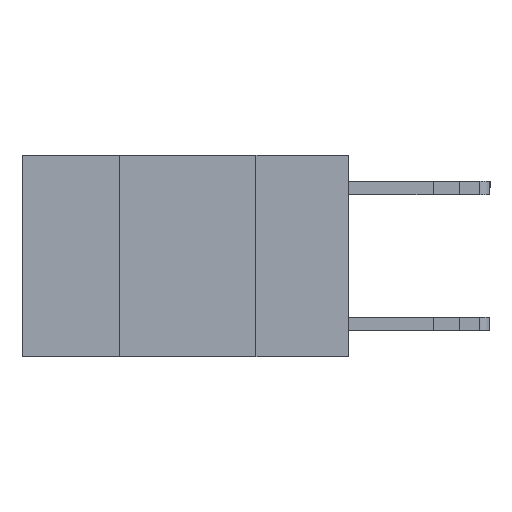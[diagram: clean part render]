
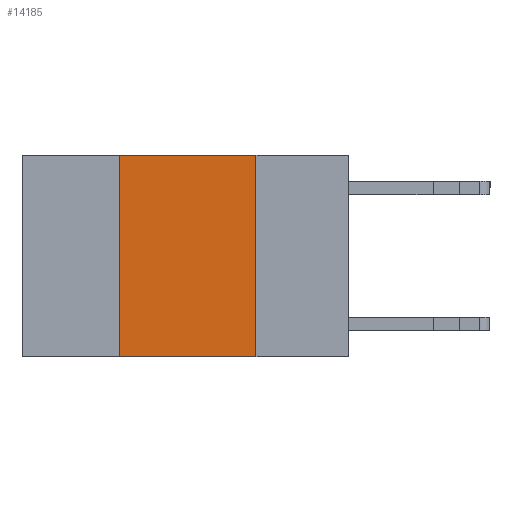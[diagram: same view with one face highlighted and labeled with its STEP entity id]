
A CAD part, left-side view. The second image highlights one B-rep face of the part: STEP entity #14185.
In plain terms, the highlighted planar face has unit normal (-1, 0, 0).
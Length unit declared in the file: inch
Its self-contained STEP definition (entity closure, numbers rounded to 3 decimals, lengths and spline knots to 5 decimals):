
#101 = EDGE_LOOP ( 'NONE', ( #18731, #4744, #9675, #9079 ) ) ;
#265 = LINE ( 'NONE', #17785, #15673 ) ;
#673 = CARTESIAN_POINT ( 'NONE',  ( 0., 0.6, -0.37 ) ) ;
#4744 = ORIENTED_EDGE ( 'NONE', *, *, #6295, .F. ) ;
#6069 = EDGE_CURVE ( 'NONE', #9672, #9356, #21163, .T. ) ;
#6085 = VECTOR ( 'NONE', #10915, 39.37008 ) ;
#6295 = EDGE_CURVE ( 'NONE', #9356, #16151, #265, .T. ) ;
#7615 = DIRECTION ( 'NONE',  ( 0., 0., -1. ) ) ;
#9074 = CARTESIAN_POINT ( 'NONE',  ( 0., 0.17, -0.37 ) ) ;
#9079 = ORIENTED_EDGE ( 'NONE', *, *, #17970, .T. ) ;
#9175 = AXIS2_PLACEMENT_3D ( 'NONE', #16132, #21436, #7615 ) ;
#9356 = VERTEX_POINT ( 'NONE', #15029 ) ;
#9433 = CARTESIAN_POINT ( 'NONE',  ( 0., 0.17, 0. ) ) ;
#9562 = VECTOR ( 'NONE', #11305, 39.37008 ) ;
#9672 = VERTEX_POINT ( 'NONE', #20808 ) ;
#9675 = ORIENTED_EDGE ( 'NONE', *, *, #6069, .F. ) ;
#9793 = VERTEX_POINT ( 'NONE', #9074 ) ;
#10817 = LINE ( 'NONE', #673, #6085 ) ;
#10915 = DIRECTION ( 'NONE',  ( 0., -1., 0. ) ) ;
#11305 = DIRECTION ( 'NONE',  ( 0., 0., 1. ) ) ;
#12551 = EDGE_CURVE ( 'NONE', #16151, #9793, #18272, .T. ) ;
#12754 = CARTESIAN_POINT ( 'NONE',  ( 0., 0.42, 0. ) ) ;
#12921 = FACE_OUTER_BOUND ( 'NONE', #101, .T. ) ;
#13404 = VECTOR ( 'NONE', #21593, 39.37008 ) ;
#14185 = ADVANCED_FACE ( 'NONE', ( #12921 ), #14686, .F. ) ;
#14686 = PLANE ( 'NONE',  #9175 ) ;
#15029 = CARTESIAN_POINT ( 'NONE',  ( 0., 0.42, 0. ) ) ;
#15673 = VECTOR ( 'NONE', #19566, 39.37008 ) ;
#16132 = CARTESIAN_POINT ( 'NONE',  ( 0., 0.6, 0. ) ) ;
#16151 = VERTEX_POINT ( 'NONE', #17762 ) ;
#17762 = CARTESIAN_POINT ( 'NONE',  ( 0., 0.17, 0. ) ) ;
#17785 = CARTESIAN_POINT ( 'NONE',  ( 0., 0.6, 0. ) ) ;
#17970 = EDGE_CURVE ( 'NONE', #9672, #9793, #10817, .T. ) ;
#18272 = LINE ( 'NONE', #9433, #13404 ) ;
#18731 = ORIENTED_EDGE ( 'NONE', *, *, #12551, .F. ) ;
#19566 = DIRECTION ( 'NONE',  ( 0., -1., 0. ) ) ;
#20808 = CARTESIAN_POINT ( 'NONE',  ( 0., 0.42, -0.37 ) ) ;
#21163 = LINE ( 'NONE', #12754, #9562 ) ;
#21436 = DIRECTION ( 'NONE',  ( 1., 0., 0. ) ) ;
#21593 = DIRECTION ( 'NONE',  ( 0., 0., -1. ) ) ;
